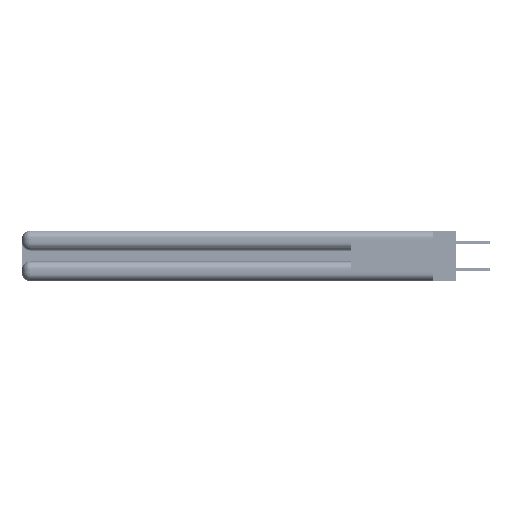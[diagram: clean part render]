
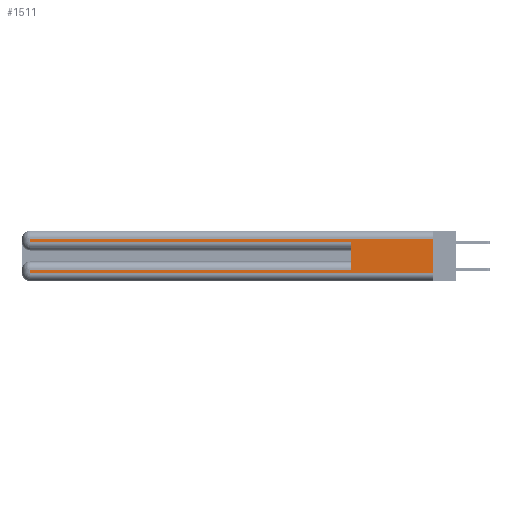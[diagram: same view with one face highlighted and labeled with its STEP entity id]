
A CAD part, left-side view. The second image highlights one B-rep face of the part: STEP entity #1511.
In plain terms, the highlighted planar face has unit normal (-1, 0, 0).
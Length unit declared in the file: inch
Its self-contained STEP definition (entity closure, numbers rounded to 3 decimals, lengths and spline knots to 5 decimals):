
#20 = CARTESIAN_POINT ( 'NONE',  ( 0., 0.6, 0.085 ) ) ;
#414 = FACE_OUTER_BOUND ( 'NONE', #20003, .T. ) ;
#734 = ORIENTED_EDGE ( 'NONE', *, *, #10912, .F. ) ;
#816 = VERTEX_POINT ( 'NONE', #22488 ) ;
#1105 = DIRECTION ( 'NONE',  ( 1., 0., 0. ) ) ;
#1511 = ADVANCED_FACE ( 'NONE', ( #414 ), #45195, .F. ) ;
#1566 = LINE ( 'NONE', #15577, #15510 ) ;
#1678 = CARTESIAN_POINT ( 'NONE',  ( 0., 0.6, 0.285 ) ) ;
#2020 = CARTESIAN_POINT ( 'NONE',  ( 0., 2.94, 0.285 ) ) ;
#4152 = EDGE_CURVE ( 'NONE', #816, #17847, #8108, .T. ) ;
#5539 = DIRECTION ( 'NONE',  ( 0., 0., 1. ) ) ;
#6299 = CARTESIAN_POINT ( 'NONE',  ( 0., 0., 0.06 ) ) ;
#6537 = VERTEX_POINT ( 'NONE', #8518 ) ;
#6765 = LINE ( 'NONE', #41182, #10975 ) ;
#7413 = CARTESIAN_POINT ( 'NONE',  ( 0., 0., 0.31 ) ) ;
#8108 = LINE ( 'NONE', #51973, #43653 ) ;
#8518 = CARTESIAN_POINT ( 'NONE',  ( 0., 0., 0.31 ) ) ;
#9301 = CARTESIAN_POINT ( 'NONE',  ( 0., 2.94, 0.37 ) ) ;
#10547 = VERTEX_POINT ( 'NONE', #30790 ) ;
#10912 = EDGE_CURVE ( 'NONE', #6537, #14788, #48970, .T. ) ;
#10975 = VECTOR ( 'NONE', #5539, 39.37008 ) ;
#14738 = AXIS2_PLACEMENT_3D ( 'NONE', #27270, #1105, #23184 ) ;
#14788 = VERTEX_POINT ( 'NONE', #6299 ) ;
#14835 = EDGE_CURVE ( 'NONE', #30208, #47824, #6765, .T. ) ;
#15510 = VECTOR ( 'NONE', #46798, 39.37008 ) ;
#15577 = CARTESIAN_POINT ( 'NONE',  ( 0., 0., 0.085 ) ) ;
#15989 = ORIENTED_EDGE ( 'NONE', *, *, #48032, .T. ) ;
#17080 = VECTOR ( 'NONE', #37850, 39.37008 ) ;
#17847 = VERTEX_POINT ( 'NONE', #2020 ) ;
#20003 = EDGE_LOOP ( 'NONE', ( #734, #36656, #20526, #35940, #22241, #51198, #15989, #23004 ) ) ;
#20526 = ORIENTED_EDGE ( 'NONE', *, *, #4152, .T. ) ;
#22241 = ORIENTED_EDGE ( 'NONE', *, *, #14835, .F. ) ;
#22488 = CARTESIAN_POINT ( 'NONE',  ( 0., 2.94, 0.31 ) ) ;
#23004 = ORIENTED_EDGE ( 'NONE', *, *, #26969, .T. ) ;
#23184 = DIRECTION ( 'NONE',  ( 0., 0., -1. ) ) ;
#26969 = EDGE_CURVE ( 'NONE', #49301, #14788, #47673, .T. ) ;
#27270 = CARTESIAN_POINT ( 'NONE',  ( 0., 0., 0.37 ) ) ;
#29068 = DIRECTION ( 'NONE',  ( 0., 1., 0. ) ) ;
#29082 = DIRECTION ( 'NONE',  ( 0., -1., 0. ) ) ;
#29560 = VECTOR ( 'NONE', #29082, 39.37008 ) ;
#30208 = VERTEX_POINT ( 'NONE', #20 ) ;
#30790 = CARTESIAN_POINT ( 'NONE',  ( 0., 2.94, 0.085 ) ) ;
#33653 = VECTOR ( 'NONE', #33658, 39.37008 ) ;
#33658 = DIRECTION ( 'NONE',  ( 0., 0., -1. ) ) ;
#33742 = CARTESIAN_POINT ( 'NONE',  ( 0., 0., 0.06 ) ) ;
#35940 = ORIENTED_EDGE ( 'NONE', *, *, #55446, .T. ) ;
#36656 = ORIENTED_EDGE ( 'NONE', *, *, #47279, .T. ) ;
#37653 = CARTESIAN_POINT ( 'NONE',  ( 0., 0., 0.285 ) ) ;
#37850 = DIRECTION ( 'NONE',  ( 0., -1., 0. ) ) ;
#41182 = CARTESIAN_POINT ( 'NONE',  ( 0., 0.6, 0.145 ) ) ;
#43012 = VECTOR ( 'NONE', #44960, 39.37008 ) ;
#43083 = LINE ( 'NONE', #7413, #56318 ) ;
#43600 = EDGE_CURVE ( 'NONE', #30208, #10547, #1566, .T. ) ;
#43653 = VECTOR ( 'NONE', #56085, 39.37008 ) ;
#44960 = DIRECTION ( 'NONE',  ( 0., 0., -1. ) ) ;
#45195 = PLANE ( 'NONE',  #14738 ) ;
#45662 = LINE ( 'NONE', #37653, #17080 ) ;
#46798 = DIRECTION ( 'NONE',  ( 0., 1., 0. ) ) ;
#46890 = CARTESIAN_POINT ( 'NONE',  ( 0., 2.94, 0.06 ) ) ;
#47279 = EDGE_CURVE ( 'NONE', #6537, #816, #43083, .T. ) ;
#47673 = LINE ( 'NONE', #33742, #29560 ) ;
#47824 = VERTEX_POINT ( 'NONE', #1678 ) ;
#48032 = EDGE_CURVE ( 'NONE', #10547, #49301, #49995, .T. ) ;
#48970 = LINE ( 'NONE', #51373, #33653 ) ;
#49301 = VERTEX_POINT ( 'NONE', #46890 ) ;
#49995 = LINE ( 'NONE', #9301, #43012 ) ;
#51198 = ORIENTED_EDGE ( 'NONE', *, *, #43600, .T. ) ;
#51373 = CARTESIAN_POINT ( 'NONE',  ( 0., 0., 0.37 ) ) ;
#51973 = CARTESIAN_POINT ( 'NONE',  ( 0., 2.94, 0.37 ) ) ;
#55446 = EDGE_CURVE ( 'NONE', #17847, #47824, #45662, .T. ) ;
#56085 = DIRECTION ( 'NONE',  ( 0., 0., -1. ) ) ;
#56318 = VECTOR ( 'NONE', #29068, 39.37008 ) ;
